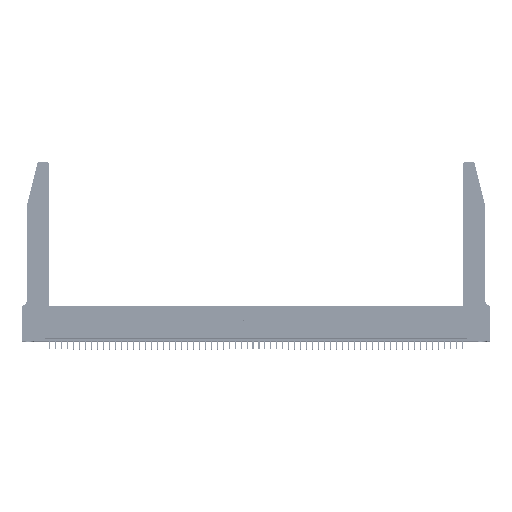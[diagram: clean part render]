
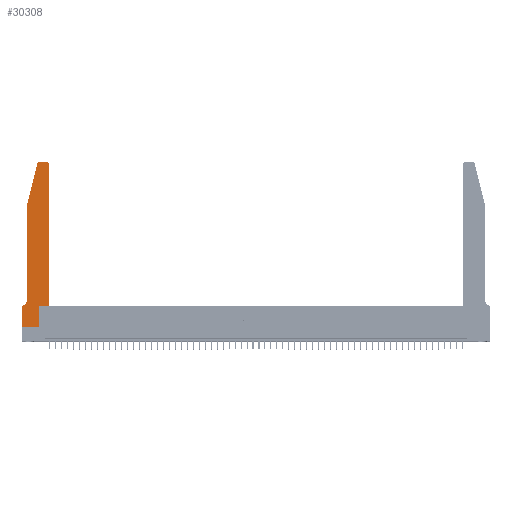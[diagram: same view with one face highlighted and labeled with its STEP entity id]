
A CAD part, top view. The second image highlights one B-rep face of the part: STEP entity #30308.
In plain terms, the highlighted planar face has unit normal (0, 0, 1).
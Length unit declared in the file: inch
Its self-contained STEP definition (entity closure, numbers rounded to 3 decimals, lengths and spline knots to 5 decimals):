
#877 = AXIS2_PLACEMENT_3D ( 'NONE', #8839, #30153, #26174 ) ;
#990 = EDGE_CURVE ( 'NONE', #21330, #26090, #6438, .T. ) ;
#2625 = EDGE_CURVE ( 'NONE', #4368, #23727, #19175, .T. ) ;
#3577 = VECTOR ( 'NONE', #47961, 39.37008 ) ;
#4264 = DIRECTION ( 'NONE',  ( -1., 0., 0. ) ) ;
#4368 = VERTEX_POINT ( 'NONE', #6993 ) ;
#4819 = AXIS2_PLACEMENT_3D ( 'NONE', #14212, #27566, #40329 ) ;
#5522 = EDGE_CURVE ( 'NONE', #50429, #23029, #17636, .T. ) ;
#6055 = LINE ( 'NONE', #27370, #23970 ) ;
#6438 = LINE ( 'NONE', #7566, #24257 ) ;
#6899 = ORIENTED_EDGE ( 'NONE', *, *, #990, .T. ) ;
#6993 = CARTESIAN_POINT ( 'NONE',  ( 0.2865, 0., 0.37 ) ) ;
#7566 = CARTESIAN_POINT ( 'NONE',  ( 0.0755, 2., 0.37 ) ) ;
#7752 = EDGE_CURVE ( 'NONE', #26090, #50429, #28676, .T. ) ;
#8822 = CARTESIAN_POINT ( 'NONE',  ( 0.0755, 0.35, 0.37 ) ) ;
#8839 = CARTESIAN_POINT ( 'NONE',  ( 0.284, 2.72, 0.37 ) ) ;
#9082 = VECTOR ( 'NONE', #46932, 39.37008 ) ;
#9097 = PLANE ( 'NONE',  #50673 ) ;
#9781 = EDGE_CURVE ( 'NONE', #47211, #45150, #49798, .T. ) ;
#11175 = CIRCLE ( 'NONE', #4819, 0.03 ) ;
#12729 = DIRECTION ( 'NONE',  ( 1., 0., 0. ) ) ;
#12774 = VECTOR ( 'NONE', #34954, 39.37008 ) ;
#13284 = EDGE_CURVE ( 'NONE', #14065, #16861, #11175, .T. ) ;
#13366 = DIRECTION ( 'NONE',  ( 1., 0., 0. ) ) ;
#14065 = VERTEX_POINT ( 'NONE', #48628 ) ;
#14212 = CARTESIAN_POINT ( 'NONE',  ( 0.4205, 2.72, 0.37 ) ) ;
#14294 = EDGE_CURVE ( 'NONE', #23029, #39027, #6055, .T. ) ;
#15404 = ORIENTED_EDGE ( 'NONE', *, *, #24338, .T. ) ;
#16095 = ORIENTED_EDGE ( 'NONE', *, *, #55756, .T. ) ;
#16861 = VERTEX_POINT ( 'NONE', #20382 ) ;
#17010 = VECTOR ( 'NONE', #4264, 39.37008 ) ;
#17161 = CARTESIAN_POINT ( 'NONE',  ( 0.4505, 0.35, 0.37 ) ) ;
#17636 = LINE ( 'NONE', #8822, #12774 ) ;
#18855 = DIRECTION ( 'NONE',  ( 0., -1., 0. ) ) ;
#19175 = LINE ( 'NONE', #48671, #21631 ) ;
#19811 = ORIENTED_EDGE ( 'NONE', *, *, #9781, .T. ) ;
#20382 = CARTESIAN_POINT ( 'NONE',  ( 0.4205, 2.75, 0.37 ) ) ;
#21330 = VERTEX_POINT ( 'NONE', #53852 ) ;
#21631 = VECTOR ( 'NONE', #49220, 39.37008 ) ;
#21794 = ORIENTED_EDGE ( 'NONE', *, *, #14294, .T. ) ;
#21891 = LINE ( 'NONE', #34945, #3577 ) ;
#22154 = CARTESIAN_POINT ( 'NONE',  ( 0.2605, 2.75, 0.37 ) ) ;
#23029 = VERTEX_POINT ( 'NONE', #39397 ) ;
#23727 = VERTEX_POINT ( 'NONE', #51429 ) ;
#23970 = VECTOR ( 'NONE', #18855, 39.37008 ) ;
#24257 = VECTOR ( 'NONE', #32301, 39.37008 ) ;
#24338 = EDGE_CURVE ( 'NONE', #26800, #14065, #21891, .T. ) ;
#25662 = LINE ( 'NONE', #33344, #54325 ) ;
#25801 = CARTESIAN_POINT ( 'NONE',  ( 0., 0., 0.37 ) ) ;
#26090 = VERTEX_POINT ( 'NONE', #50357 ) ;
#26124 = LINE ( 'NONE', #22154, #17010 ) ;
#26174 = DIRECTION ( 'NONE',  ( 1., 0., 0. ) ) ;
#26789 = EDGE_LOOP ( 'NONE', ( #44189, #19811, #16095, #6899, #54303, #52787, #21794, #50904, #37766, #49901, #15404, #45921 ) ) ;
#26800 = VERTEX_POINT ( 'NONE', #47445 ) ;
#27370 = CARTESIAN_POINT ( 'NONE',  ( 0., 0., 0.37 ) ) ;
#27566 = DIRECTION ( 'NONE',  ( 0., 0., 1. ) ) ;
#27732 = AXIS2_PLACEMENT_3D ( 'NONE', #49998, #54527, #31889 ) ;
#28676 = CIRCLE ( 'NONE', #27732, 0.07 ) ;
#29213 = LINE ( 'NONE', #25801, #30315 ) ;
#29653 = LINE ( 'NONE', #17161, #9082 ) ;
#30153 = DIRECTION ( 'NONE',  ( 0., 0., 1. ) ) ;
#30308 = ADVANCED_FACE ( 'NONE', ( #38662 ), #9097, .T. ) ;
#30315 = VECTOR ( 'NONE', #12729, 39.37008 ) ;
#31621 = EDGE_CURVE ( 'NONE', #23727, #26800, #29653, .T. ) ;
#31889 = DIRECTION ( 'NONE',  ( -1., 0., 0. ) ) ;
#32301 = DIRECTION ( 'NONE',  ( 0., -1., 0. ) ) ;
#33344 = CARTESIAN_POINT ( 'NONE',  ( 0.0755, 2., 0.37 ) ) ;
#34945 = CARTESIAN_POINT ( 'NONE',  ( 0.4505, 0.35, 0.37 ) ) ;
#34954 = DIRECTION ( 'NONE',  ( -1., 0., 0. ) ) ;
#37766 = ORIENTED_EDGE ( 'NONE', *, *, #2625, .T. ) ;
#38662 = FACE_OUTER_BOUND ( 'NONE', #26789, .T. ) ;
#39027 = VERTEX_POINT ( 'NONE', #48930 ) ;
#39217 = DIRECTION ( 'NONE',  ( 0., 0., 1. ) ) ;
#39397 = CARTESIAN_POINT ( 'NONE',  ( 0., 0.35, 0.37 ) ) ;
#40329 = DIRECTION ( 'NONE',  ( 1., 0., 0. ) ) ;
#43801 = CARTESIAN_POINT ( 'NONE',  ( 0.284, 2.75, 0.37 ) ) ;
#44189 = ORIENTED_EDGE ( 'NONE', *, *, #52650, .T. ) ;
#45150 = VERTEX_POINT ( 'NONE', #54700 ) ;
#45921 = ORIENTED_EDGE ( 'NONE', *, *, #13284, .T. ) ;
#46139 = EDGE_CURVE ( 'NONE', #39027, #4368, #29213, .T. ) ;
#46638 = DIRECTION ( 'NONE',  ( -0.239, -0.971, 0. ) ) ;
#46932 = DIRECTION ( 'NONE',  ( 1., 0., 0. ) ) ;
#47211 = VERTEX_POINT ( 'NONE', #43801 ) ;
#47445 = CARTESIAN_POINT ( 'NONE',  ( 0.4505, 0.35, 0.37 ) ) ;
#47961 = DIRECTION ( 'NONE',  ( 0., 1., 0. ) ) ;
#48628 = CARTESIAN_POINT ( 'NONE',  ( 0.4505, 2.72, 0.37 ) ) ;
#48671 = CARTESIAN_POINT ( 'NONE',  ( 0.2865, 0.35, 0.37 ) ) ;
#48930 = CARTESIAN_POINT ( 'NONE',  ( 0., 0., 0.37 ) ) ;
#49166 = CARTESIAN_POINT ( 'NONE',  ( 0.0055, 0.35, 0.37 ) ) ;
#49220 = DIRECTION ( 'NONE',  ( 0., 1., 0. ) ) ;
#49798 = CIRCLE ( 'NONE', #877, 0.03 ) ;
#49901 = ORIENTED_EDGE ( 'NONE', *, *, #31621, .T. ) ;
#49998 = CARTESIAN_POINT ( 'NONE',  ( 0.0055, 0.42, 0.37 ) ) ;
#50357 = CARTESIAN_POINT ( 'NONE',  ( 0.0755, 0.42, 0.37 ) ) ;
#50429 = VERTEX_POINT ( 'NONE', #49166 ) ;
#50673 = AXIS2_PLACEMENT_3D ( 'NONE', #55620, #39217, #13366 ) ;
#50904 = ORIENTED_EDGE ( 'NONE', *, *, #46139, .T. ) ;
#51429 = CARTESIAN_POINT ( 'NONE',  ( 0.2865, 0.35, 0.37 ) ) ;
#52650 = EDGE_CURVE ( 'NONE', #16861, #47211, #26124, .T. ) ;
#52787 = ORIENTED_EDGE ( 'NONE', *, *, #5522, .T. ) ;
#53852 = CARTESIAN_POINT ( 'NONE',  ( 0.0755, 2., 0.37 ) ) ;
#54303 = ORIENTED_EDGE ( 'NONE', *, *, #7752, .T. ) ;
#54325 = VECTOR ( 'NONE', #46638, 39.37008 ) ;
#54527 = DIRECTION ( 'NONE',  ( 0., 0., -1. ) ) ;
#54700 = CARTESIAN_POINT ( 'NONE',  ( 0.25487, 2.72718, 0.37 ) ) ;
#55620 = CARTESIAN_POINT ( 'NONE',  ( 0., 0.35, 0.37 ) ) ;
#55756 = EDGE_CURVE ( 'NONE', #45150, #21330, #25662, .T. ) ;
